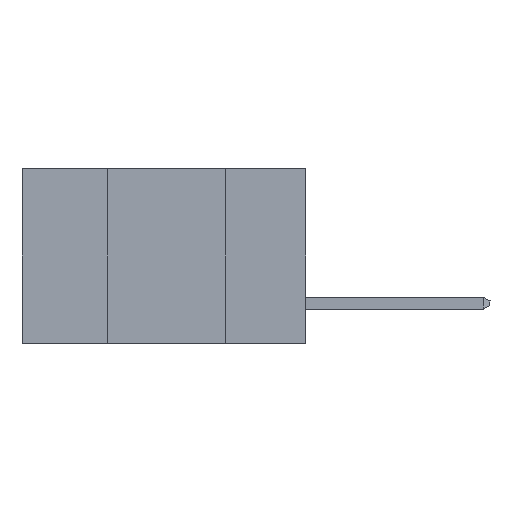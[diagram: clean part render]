
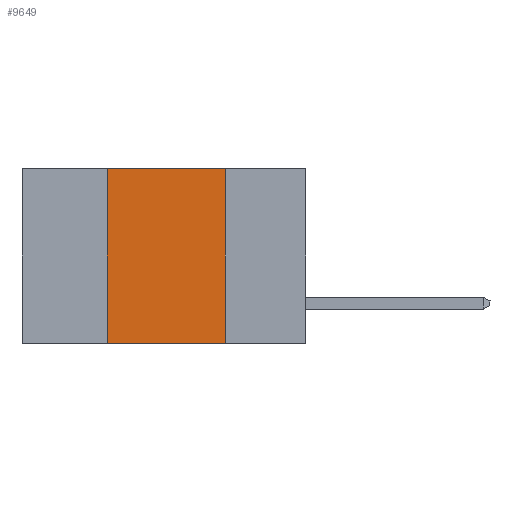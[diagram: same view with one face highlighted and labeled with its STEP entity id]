
A CAD part, left-side view. The second image highlights one B-rep face of the part: STEP entity #9649.
In plain terms, the highlighted planar face has unit normal (-1, 0, 0).
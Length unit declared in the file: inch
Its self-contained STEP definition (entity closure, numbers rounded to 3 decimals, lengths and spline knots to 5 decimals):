
#676 = DIRECTION ( 'NONE',  ( 0., -1., 0. ) ) ;
#1283 = CARTESIAN_POINT ( 'NONE',  ( 0., 0.6, 0. ) ) ;
#2664 = CARTESIAN_POINT ( 'NONE',  ( 0., 0.6, -0.37 ) ) ;
#3450 = DIRECTION ( 'NONE',  ( 0., 0., -1. ) ) ;
#3528 = VECTOR ( 'NONE', #16434, 39.37008 ) ;
#4694 = CARTESIAN_POINT ( 'NONE',  ( 0., 0.17, 0. ) ) ;
#5046 = DIRECTION ( 'NONE',  ( 0., -1., 0. ) ) ;
#5407 = EDGE_CURVE ( 'NONE', #21690, #11582, #16200, .T. ) ;
#5565 = LINE ( 'NONE', #15859, #11123 ) ;
#9649 = ADVANCED_FACE ( 'NONE', ( #11743 ), #22297, .F. ) ;
#10161 = VERTEX_POINT ( 'NONE', #30508 ) ;
#10208 = ORIENTED_EDGE ( 'NONE', *, *, #21051, .F. ) ;
#11123 = VECTOR ( 'NONE', #18251, 39.37008 ) ;
#11582 = VERTEX_POINT ( 'NONE', #13497 ) ;
#11739 = CARTESIAN_POINT ( 'NONE',  ( 0., 0.42, 0. ) ) ;
#11743 = FACE_OUTER_BOUND ( 'NONE', #23272, .T. ) ;
#12498 = CARTESIAN_POINT ( 'NONE',  ( 0., 0.6, 0. ) ) ;
#13356 = VERTEX_POINT ( 'NONE', #4694 ) ;
#13497 = CARTESIAN_POINT ( 'NONE',  ( 0., 0.42, 0. ) ) ;
#15260 = VECTOR ( 'NONE', #5046, 39.37008 ) ;
#15342 = ORIENTED_EDGE ( 'NONE', *, *, #22323, .F. ) ;
#15466 = ORIENTED_EDGE ( 'NONE', *, *, #22122, .T. ) ;
#15859 = CARTESIAN_POINT ( 'NONE',  ( 0., 0.17, 0. ) ) ;
#16200 = LINE ( 'NONE', #11739, #3528 ) ;
#16434 = DIRECTION ( 'NONE',  ( 0., 0., 1. ) ) ;
#17568 = LINE ( 'NONE', #12498, #27138 ) ;
#17969 = ORIENTED_EDGE ( 'NONE', *, *, #5407, .F. ) ;
#18251 = DIRECTION ( 'NONE',  ( 0., 0., -1. ) ) ;
#21051 = EDGE_CURVE ( 'NONE', #11582, #13356, #17568, .T. ) ;
#21396 = AXIS2_PLACEMENT_3D ( 'NONE', #1283, #22697, #3450 ) ;
#21690 = VERTEX_POINT ( 'NONE', #23024 ) ;
#22122 = EDGE_CURVE ( 'NONE', #21690, #10161, #22690, .T. ) ;
#22297 = PLANE ( 'NONE',  #21396 ) ;
#22323 = EDGE_CURVE ( 'NONE', #13356, #10161, #5565, .T. ) ;
#22690 = LINE ( 'NONE', #2664, #15260 ) ;
#22697 = DIRECTION ( 'NONE',  ( 1., 0., 0. ) ) ;
#23024 = CARTESIAN_POINT ( 'NONE',  ( 0., 0.42, -0.37 ) ) ;
#23272 = EDGE_LOOP ( 'NONE', ( #15342, #10208, #17969, #15466 ) ) ;
#27138 = VECTOR ( 'NONE', #676, 39.37008 ) ;
#30508 = CARTESIAN_POINT ( 'NONE',  ( 0., 0.17, -0.37 ) ) ;
